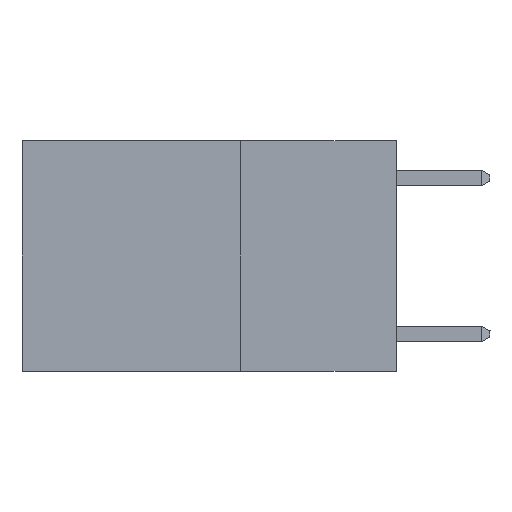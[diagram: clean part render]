
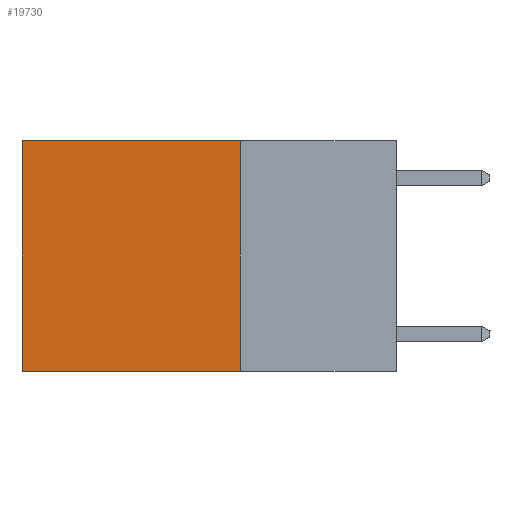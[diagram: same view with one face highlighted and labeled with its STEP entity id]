
A CAD part, left-side view. The second image highlights one B-rep face of the part: STEP entity #19730.
In plain terms, the highlighted planar face has unit normal (-1, 0, 0).
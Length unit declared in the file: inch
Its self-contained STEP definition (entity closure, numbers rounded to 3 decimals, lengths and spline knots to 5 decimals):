
#409 = CARTESIAN_POINT ( 'NONE',  ( 0.2625, 0.6, 0. ) ) ;
#462 = PLANE ( 'NONE',  #14447 ) ;
#694 = DIRECTION ( 'NONE',  ( 0., 1., 0. ) ) ;
#759 = VECTOR ( 'NONE', #694, 39.37008 ) ;
#1339 = CARTESIAN_POINT ( 'NONE',  ( 0.2625, 0.25, -0.37 ) ) ;
#1788 = EDGE_CURVE ( 'NONE', #15203, #23764, #20277, .T. ) ;
#3580 = DIRECTION ( 'NONE',  ( 0., 1., 0. ) ) ;
#4904 = DIRECTION ( 'NONE',  ( 0., 0., -1. ) ) ;
#5787 = EDGE_CURVE ( 'NONE', #23764, #26874, #10646, .T. ) ;
#7183 = CARTESIAN_POINT ( 'NONE',  ( 0.2625, 0.25, 0. ) ) ;
#8767 = ORIENTED_EDGE ( 'NONE', *, *, #19128, .T. ) ;
#10332 = CARTESIAN_POINT ( 'NONE',  ( 0.2625, 0.25, 0. ) ) ;
#10444 = VECTOR ( 'NONE', #3580, 39.37008 ) ;
#10646 = LINE ( 'NONE', #1339, #10444 ) ;
#11337 = VERTEX_POINT ( 'NONE', #20002 ) ;
#11678 = LINE ( 'NONE', #409, #27582 ) ;
#11711 = CARTESIAN_POINT ( 'NONE',  ( 0.2625, 0.25, 0. ) ) ;
#11741 = ORIENTED_EDGE ( 'NONE', *, *, #5787, .F. ) ;
#13226 = ORIENTED_EDGE ( 'NONE', *, *, #20320, .T. ) ;
#13510 = CARTESIAN_POINT ( 'NONE',  ( 0.2625, 0.6, -0.37 ) ) ;
#13738 = DIRECTION ( 'NONE',  ( 0., 0., -1. ) ) ;
#14447 = AXIS2_PLACEMENT_3D ( 'NONE', #7183, #26216, #13738 ) ;
#14965 = CARTESIAN_POINT ( 'NONE',  ( 0.2625, 0.25, 0. ) ) ;
#15203 = VERTEX_POINT ( 'NONE', #14965 ) ;
#18139 = LINE ( 'NONE', #11711, #759 ) ;
#18629 = CARTESIAN_POINT ( 'NONE',  ( 0.2625, 0.25, -0.37 ) ) ;
#19128 = EDGE_CURVE ( 'NONE', #15203, #11337, #18139, .T. ) ;
#19453 = VECTOR ( 'NONE', #25023, 39.37008 ) ;
#19730 = ADVANCED_FACE ( 'NONE', ( #19731 ), #462, .F. ) ;
#19731 = FACE_OUTER_BOUND ( 'NONE', #22153, .T. ) ;
#20002 = CARTESIAN_POINT ( 'NONE',  ( 0.2625, 0.6, 0. ) ) ;
#20277 = LINE ( 'NONE', #10332, #19453 ) ;
#20320 = EDGE_CURVE ( 'NONE', #11337, #26874, #11678, .T. ) ;
#22153 = EDGE_LOOP ( 'NONE', ( #13226, #11741, #25311, #8767 ) ) ;
#23764 = VERTEX_POINT ( 'NONE', #18629 ) ;
#25023 = DIRECTION ( 'NONE',  ( 0., 0., -1. ) ) ;
#25311 = ORIENTED_EDGE ( 'NONE', *, *, #1788, .F. ) ;
#26216 = DIRECTION ( 'NONE',  ( 1., 0., 0. ) ) ;
#26874 = VERTEX_POINT ( 'NONE', #13510 ) ;
#27582 = VECTOR ( 'NONE', #4904, 39.37008 ) ;
